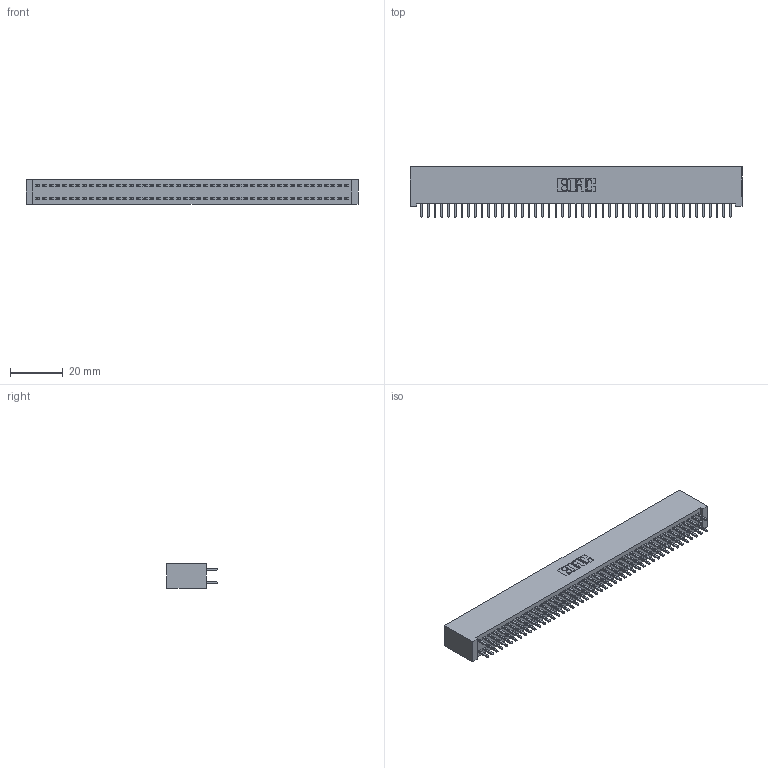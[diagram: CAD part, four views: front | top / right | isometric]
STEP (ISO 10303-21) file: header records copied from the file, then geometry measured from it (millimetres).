
FILE_DESCRIPTION (( 'STEP AP203' ), '1' );
FILE_NAME ('392-094-521-201.STEP', '2019-10-09T19:13:14', ( '' ), ( '' ), 'SwSTEP 2.0', 'SolidWorks 2016', '' );
FILE_SCHEMA (( 'CONFIG_CONTROL_DESIGN' ));
Length unit declared in the file: inch
Products named in the file (3): 342 Part_Lugless; 345-292-001_345-293-121; 392-094-521-201
Assembly tree (95 placements, depth 2):
  392-094-521-201
    342 Part_Lugless
    345-292-001_345-293-121  x94
Bounding box: 125.63 x 19.06 x 9.4 mm (x, y, z)
Volume: 11712.5 mm3; surface area: 19374.7 mm2
Topology: 95 solids, 95 shells, 4990 faces, 14845 edges, 9770 vertices
Faces by surface type: plane 3446, cylinder 1544
Entity records: 29199 total; most frequent: CARTESIAN_POINT 4830, ORIENTED_EDGE 4766, DIRECTION 4111, EDGE_CURVE 2383, VECTOR 2263, LINE 2263, VERTEX_POINT 1586, AXIS2_PLACEMENT_3D 924
